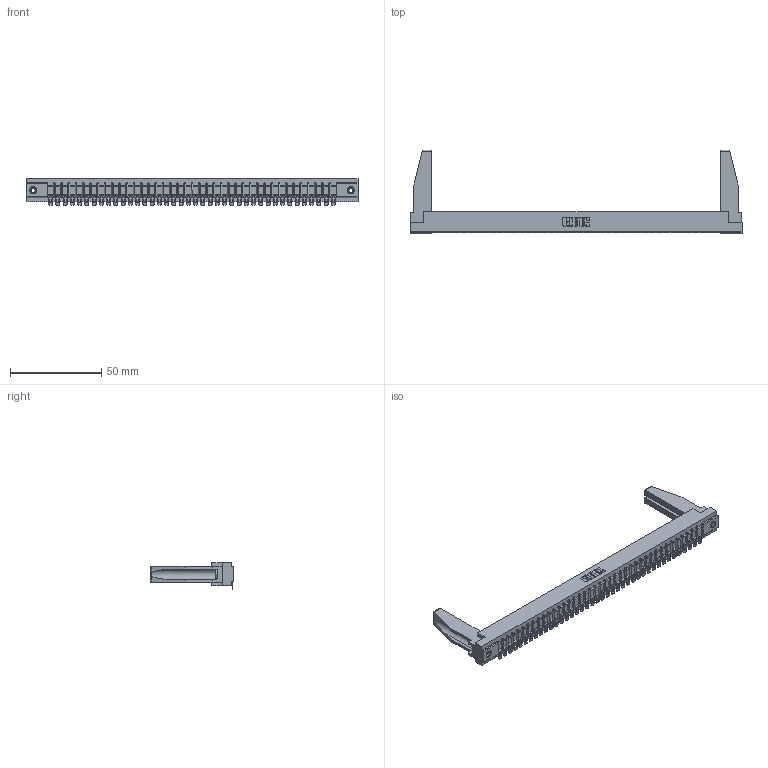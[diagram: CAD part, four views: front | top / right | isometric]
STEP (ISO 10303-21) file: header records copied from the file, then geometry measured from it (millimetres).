
FILE_DESCRIPTION (( 'STEP AP203' ), '1' );
FILE_NAME ('357-040-454-178.STEP', '2020-10-03T06:44:00', ( '' ), ( '' ), 'SwSTEP 2.0', 'SolidWorks 2020', '' );
FILE_SCHEMA (( 'CONFIG_CONTROL_DESIGN' ));
Length unit declared in the file: inch
Products named in the file (5): 307-220-078; 307 Part_.156 Dia Mounting Holes; 345-250-001_345-250-001-102; 357-040-454-178; 307-290-002_554
Assembly tree (45 placements, depth 2):
  357-040-454-178
    307 Part_.156 Dia Mounting Holes
    307-290-002_554  x40
    307-220-078  x2
    345-250-001_345-250-001-102  x2
Bounding box: 181.51 x 45.72 x 14.52 mm (x, y, z)
Volume: 23416.5 mm3; surface area: 28357.4 mm2
Topology: 45 solids, 45 shells, 3529 faces, 10773 edges, 7062 vertices
Faces by surface type: plane 1994, cylinder 1437, sphere 82, cone 12, torus 4
Entity records: 37942 total; most frequent: CARTESIAN_POINT 6400, ORIENTED_EDGE 6346, DIRECTION 6181, EDGE_CURVE 3173, LINE 2427, VECTOR 2427, VERTEX_POINT 2054, AXIS2_PLACEMENT_3D 1877
